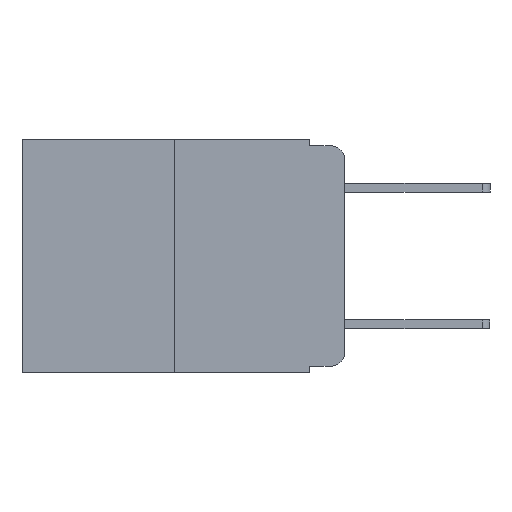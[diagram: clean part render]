
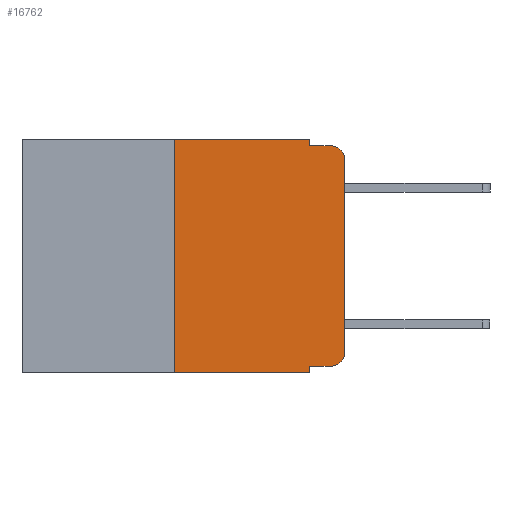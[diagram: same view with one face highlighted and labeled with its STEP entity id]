
A CAD part, left-side view. The second image highlights one B-rep face of the part: STEP entity #16762.
In plain terms, the highlighted planar face has unit normal (-1, 0, 0).
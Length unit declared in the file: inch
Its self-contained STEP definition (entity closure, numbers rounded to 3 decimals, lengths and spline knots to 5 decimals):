
#247 = FACE_OUTER_BOUND ( 'NONE', #22919, .T. ) ;
#318 = CARTESIAN_POINT ( 'NONE',  ( 0., 0.051, -0.333 ) ) ;
#777 = CARTESIAN_POINT ( 'NONE',  ( 0., 0.051, 0. ) ) ;
#1015 = ORIENTED_EDGE ( 'NONE', *, *, #17364, .T. ) ;
#1789 = VECTOR ( 'NONE', #17121, 39.37008 ) ;
#1815 = VECTOR ( 'NONE', #22963, 39.37008 ) ;
#1956 = EDGE_CURVE ( 'NONE', #6635, #24309, #17892, .T. ) ;
#2103 = CARTESIAN_POINT ( 'NONE',  ( 0., 0.051, -0.01 ) ) ;
#2443 = LINE ( 'NONE', #10227, #1815 ) ;
#2501 = CARTESIAN_POINT ( 'NONE',  ( 0., 0.051, 0. ) ) ;
#2703 = DIRECTION ( 'NONE',  ( 0., 0., -1. ) ) ;
#3275 = ORIENTED_EDGE ( 'NONE', *, *, #17782, .F. ) ;
#3359 = ORIENTED_EDGE ( 'NONE', *, *, #6015, .T. ) ;
#3508 = CARTESIAN_POINT ( 'NONE',  ( 0., 0.051, -0.343 ) ) ;
#3580 = VERTEX_POINT ( 'NONE', #14663 ) ;
#3691 = ORIENTED_EDGE ( 'NONE', *, *, #9730, .T. ) ;
#3994 = CARTESIAN_POINT ( 'NONE',  ( 0., 0.051, 0. ) ) ;
#4003 = VECTOR ( 'NONE', #19310, 39.37008 ) ;
#4008 = AXIS2_PLACEMENT_3D ( 'NONE', #9783, #22522, #11627 ) ;
#4339 = CARTESIAN_POINT ( 'NONE',  ( 0., 0.473, 0. ) ) ;
#4698 = VECTOR ( 'NONE', #15505, 39.37008 ) ;
#4905 = LINE ( 'NONE', #6237, #13745 ) ;
#4910 = VECTOR ( 'NONE', #22545, 39.37008 ) ;
#5551 = LINE ( 'NONE', #11569, #4910 ) ;
#6015 = EDGE_CURVE ( 'NONE', #16209, #20560, #17325, .T. ) ;
#6237 = CARTESIAN_POINT ( 'NONE',  ( 0., 0.25, 0. ) ) ;
#6635 = VERTEX_POINT ( 'NONE', #9914 ) ;
#6839 = VERTEX_POINT ( 'NONE', #777 ) ;
#7010 = ORIENTED_EDGE ( 'NONE', *, *, #17333, .T. ) ;
#8305 = LINE ( 'NONE', #3994, #1789 ) ;
#8557 = ORIENTED_EDGE ( 'NONE', *, *, #9821, .T. ) ;
#8676 = VECTOR ( 'NONE', #2703, 39.37008 ) ;
#9730 = EDGE_CURVE ( 'NONE', #10294, #24309, #5551, .T. ) ;
#9783 = CARTESIAN_POINT ( 'NONE',  ( 0., 0.02, -0.313 ) ) ;
#9821 = EDGE_CURVE ( 'NONE', #6635, #16209, #17471, .T. ) ;
#9914 = CARTESIAN_POINT ( 'NONE',  ( 0., 0.051, -0.333 ) ) ;
#10214 = ORIENTED_EDGE ( 'NONE', *, *, #21632, .F. ) ;
#10227 = CARTESIAN_POINT ( 'NONE',  ( 0., 0., 0. ) ) ;
#10294 = VERTEX_POINT ( 'NONE', #19120 ) ;
#10378 = DIRECTION ( 'NONE',  ( -1., 0., 0. ) ) ;
#10863 = VERTEX_POINT ( 'NONE', #20572 ) ;
#11569 = CARTESIAN_POINT ( 'NONE',  ( 0., 0.473, -0.343 ) ) ;
#11627 = DIRECTION ( 'NONE',  ( 0., 0., -1. ) ) ;
#11648 = ORIENTED_EDGE ( 'NONE', *, *, #17903, .F. ) ;
#11888 = CARTESIAN_POINT ( 'NONE',  ( 0., 0., -0.313 ) ) ;
#12354 = CARTESIAN_POINT ( 'NONE',  ( 0., 0.02, -0.333 ) ) ;
#12502 = DIRECTION ( 'NONE',  ( 0., 0., -1. ) ) ;
#13745 = VECTOR ( 'NONE', #19921, 39.37008 ) ;
#14663 = CARTESIAN_POINT ( 'NONE',  ( 0., 0., -0.03 ) ) ;
#14926 = ORIENTED_EDGE ( 'NONE', *, *, #18598, .F. ) ;
#15505 = DIRECTION ( 'NONE',  ( 0., -1., 0. ) ) ;
#15657 = DIRECTION ( 'NONE',  ( 0., -1., 0. ) ) ;
#15796 = CIRCLE ( 'NONE', #23569, 0.02 ) ;
#16120 = CARTESIAN_POINT ( 'NONE',  ( 0., 0.473, 0. ) ) ;
#16209 = VERTEX_POINT ( 'NONE', #12354 ) ;
#16762 = ADVANCED_FACE ( 'NONE', ( #247 ), #17987, .F. ) ;
#17121 = DIRECTION ( 'NONE',  ( 0., 0., -1. ) ) ;
#17325 = CIRCLE ( 'NONE', #4008, 0.02 ) ;
#17333 = EDGE_CURVE ( 'NONE', #20560, #3580, #2443, .T. ) ;
#17364 = EDGE_CURVE ( 'NONE', #3580, #10863, #15796, .T. ) ;
#17415 = CARTESIAN_POINT ( 'NONE',  ( 0., 0.051, -0.01 ) ) ;
#17471 = LINE ( 'NONE', #318, #22267 ) ;
#17782 = EDGE_CURVE ( 'NONE', #6839, #18986, #8305, .T. ) ;
#17892 = LINE ( 'NONE', #2501, #8676 ) ;
#17903 = EDGE_CURVE ( 'NONE', #23302, #6839, #18965, .T. ) ;
#17987 = PLANE ( 'NONE',  #23250 ) ;
#18598 = EDGE_CURVE ( 'NONE', #10294, #23302, #4905, .T. ) ;
#18965 = LINE ( 'NONE', #4339, #4003 ) ;
#18986 = VERTEX_POINT ( 'NONE', #17415 ) ;
#19120 = CARTESIAN_POINT ( 'NONE',  ( 0., 0.25, -0.343 ) ) ;
#19310 = DIRECTION ( 'NONE',  ( 0., -1., 0. ) ) ;
#19594 = LINE ( 'NONE', #2103, #4698 ) ;
#19921 = DIRECTION ( 'NONE',  ( 0., 0., 1. ) ) ;
#20560 = VERTEX_POINT ( 'NONE', #11888 ) ;
#20572 = CARTESIAN_POINT ( 'NONE',  ( 0., 0.02, -0.01 ) ) ;
#20780 = CARTESIAN_POINT ( 'NONE',  ( 0., 0.25, 0. ) ) ;
#21343 = CARTESIAN_POINT ( 'NONE',  ( 0., 0.02, -0.03 ) ) ;
#21632 = EDGE_CURVE ( 'NONE', #18986, #10863, #19594, .T. ) ;
#22267 = VECTOR ( 'NONE', #15657, 39.37008 ) ;
#22522 = DIRECTION ( 'NONE',  ( -1., 0., 0. ) ) ;
#22545 = DIRECTION ( 'NONE',  ( 0., -1., 0. ) ) ;
#22919 = EDGE_LOOP ( 'NONE', ( #7010, #1015, #10214, #3275, #11648, #14926, #3691, #24218, #8557, #3359 ) ) ;
#22963 = DIRECTION ( 'NONE',  ( 0., 0., 1. ) ) ;
#23111 = DIRECTION ( 'NONE',  ( 0., 0., -1. ) ) ;
#23250 = AXIS2_PLACEMENT_3D ( 'NONE', #16120, #23387, #12502 ) ;
#23302 = VERTEX_POINT ( 'NONE', #20780 ) ;
#23387 = DIRECTION ( 'NONE',  ( 1., 0., 0. ) ) ;
#23569 = AXIS2_PLACEMENT_3D ( 'NONE', #21343, #10378, #23111 ) ;
#24218 = ORIENTED_EDGE ( 'NONE', *, *, #1956, .F. ) ;
#24309 = VERTEX_POINT ( 'NONE', #3508 ) ;
